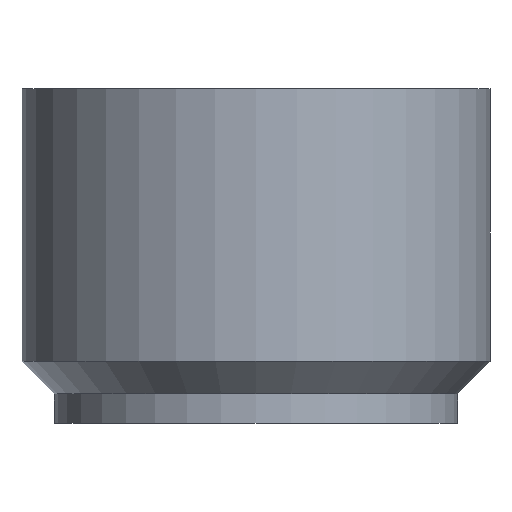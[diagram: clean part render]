
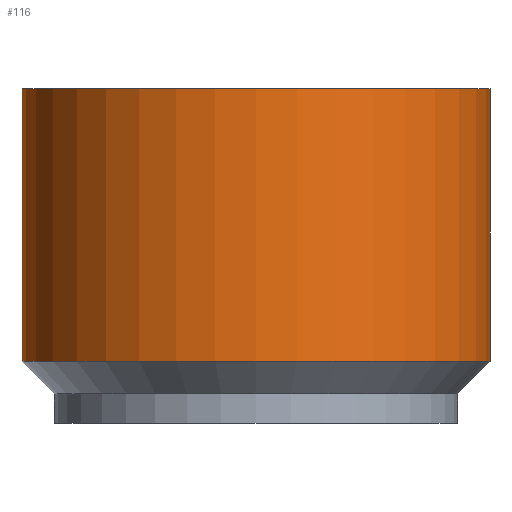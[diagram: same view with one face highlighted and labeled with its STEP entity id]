
A CAD part, left-side view. The second image highlights one B-rep face of the part: STEP entity #116.
In plain terms, the highlighted cylindrical face has radius 25.146 mm (diameter 50.292 mm), a partial arc.
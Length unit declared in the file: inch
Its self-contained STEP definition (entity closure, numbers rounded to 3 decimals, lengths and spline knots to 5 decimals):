
#67 = CARTESIAN_POINT ( 'NONE',  ( 0., -0.99, 0.66667 ) ) ;
#68 = ORIENTED_EDGE ( 'NONE', *, *, #507, .F. ) ;
#80 = CARTESIAN_POINT ( 'NONE',  ( 0., -0.99, 0.2625 ) ) ;
#95 = CARTESIAN_POINT ( 'NONE',  ( 0., 0., 0.66667 ) ) ;
#102 = DIRECTION ( 'NONE',  ( 0., 1., 0. ) ) ;
#116 = ADVANCED_FACE ( 'NONE', ( #545 ), #844, .T. ) ;
#140 = AXIS2_PLACEMENT_3D ( 'NONE', #793, #318, #225 ) ;
#147 = CARTESIAN_POINT ( 'NONE',  ( 0., 0.99, 0.66667 ) ) ;
#164 = CIRCLE ( 'NONE', #241, 0.99 ) ;
#202 = VECTOR ( 'NONE', #300, 39.37008 ) ;
#204 = VERTEX_POINT ( 'NONE', #914 ) ;
#225 = DIRECTION ( 'NONE',  ( 0., 1., 0. ) ) ;
#237 = VERTEX_POINT ( 'NONE', #765 ) ;
#241 = AXIS2_PLACEMENT_3D ( 'NONE', #396, #952, #319 ) ;
#242 = CIRCLE ( 'NONE', #140, 0.99 ) ;
#293 = ORIENTED_EDGE ( 'NONE', *, *, #722, .T. ) ;
#300 = DIRECTION ( 'NONE',  ( 0., 0., -1. ) ) ;
#318 = DIRECTION ( 'NONE',  ( 0., 0., -1. ) ) ;
#319 = DIRECTION ( 'NONE',  ( 0., 1., 0. ) ) ;
#396 = CARTESIAN_POINT ( 'NONE',  ( 0., 0., 1.41667 ) ) ;
#424 = ORIENTED_EDGE ( 'NONE', *, *, #442, .T. ) ;
#442 = EDGE_CURVE ( 'NONE', #760, #237, #164, .T. ) ;
#501 = DIRECTION ( 'NONE',  ( 0., 0., -1. ) ) ;
#507 = EDGE_CURVE ( 'NONE', #760, #981, #516, .T. ) ;
#516 = LINE ( 'NONE', #67, #202 ) ;
#540 = LINE ( 'NONE', #147, #615 ) ;
#545 = FACE_OUTER_BOUND ( 'NONE', #588, .T. ) ;
#588 = EDGE_LOOP ( 'NONE', ( #68, #424, #293, #1020 ) ) ;
#615 = VECTOR ( 'NONE', #708, 39.37008 ) ;
#672 = CARTESIAN_POINT ( 'NONE',  ( 0., -0.99, 1.41667 ) ) ;
#708 = DIRECTION ( 'NONE',  ( 0., 0., -1. ) ) ;
#722 = EDGE_CURVE ( 'NONE', #237, #204, #540, .T. ) ;
#760 = VERTEX_POINT ( 'NONE', #672 ) ;
#765 = CARTESIAN_POINT ( 'NONE',  ( 0., 0.99, 1.41667 ) ) ;
#793 = CARTESIAN_POINT ( 'NONE',  ( 0., 0., 0.2625 ) ) ;
#844 = CYLINDRICAL_SURFACE ( 'NONE', #922, 0.99 ) ;
#914 = CARTESIAN_POINT ( 'NONE',  ( 0., 0.99, 0.2625 ) ) ;
#922 = AXIS2_PLACEMENT_3D ( 'NONE', #95, #501, #102 ) ;
#952 = DIRECTION ( 'NONE',  ( 0., 0., -1. ) ) ;
#981 = VERTEX_POINT ( 'NONE', #80 ) ;
#1004 = EDGE_CURVE ( 'NONE', #981, #204, #242, .T. ) ;
#1020 = ORIENTED_EDGE ( 'NONE', *, *, #1004, .F. ) ;
